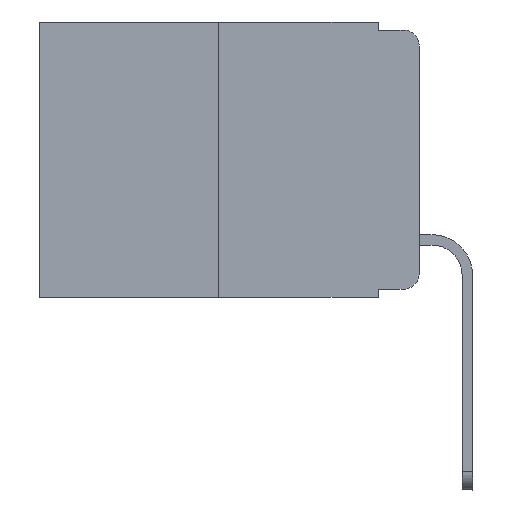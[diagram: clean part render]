
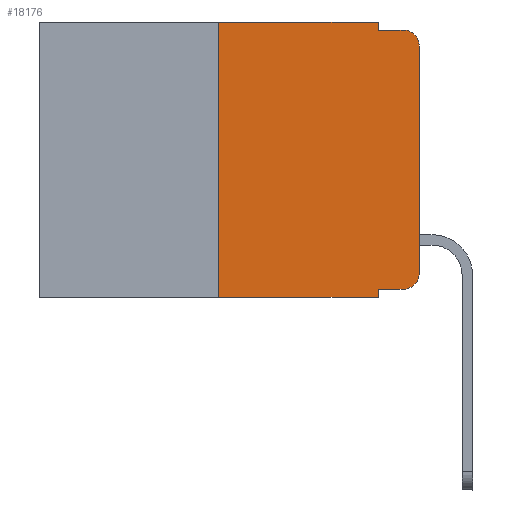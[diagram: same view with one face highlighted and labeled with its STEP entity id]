
A CAD part, left-side view. The second image highlights one B-rep face of the part: STEP entity #18176.
In plain terms, the highlighted planar face has unit normal (-1, 0, 0).
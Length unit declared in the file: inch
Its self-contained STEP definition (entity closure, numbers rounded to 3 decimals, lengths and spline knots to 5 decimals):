
#63 = LINE ( 'NONE', #7052, #14666 ) ;
#671 = EDGE_CURVE ( 'NONE', #14336, #9487, #5122, .T. ) ;
#809 = CARTESIAN_POINT ( 'NONE',  ( 0., 0.051, -0.01 ) ) ;
#1012 = AXIS2_PLACEMENT_3D ( 'NONE', #3550, #15054, #13811 ) ;
#1521 = EDGE_CURVE ( 'NONE', #14336, #9455, #9280, .T. ) ;
#2181 = CARTESIAN_POINT ( 'NONE',  ( 0., 0.473, -0.343 ) ) ;
#2260 = CARTESIAN_POINT ( 'NONE',  ( 0., 0.25, 0. ) ) ;
#2397 = EDGE_CURVE ( 'NONE', #13521, #18033, #18646, .T. ) ;
#2417 = CARTESIAN_POINT ( 'NONE',  ( 0., 0.02, -0.313 ) ) ;
#2476 = EDGE_CURVE ( 'NONE', #17727, #13521, #7102, .T. ) ;
#2742 = DIRECTION ( 'NONE',  ( 0., 0., -1. ) ) ;
#3067 = CARTESIAN_POINT ( 'NONE',  ( 0., 0., 0. ) ) ;
#3352 = CARTESIAN_POINT ( 'NONE',  ( 0., 0.02, -0.03 ) ) ;
#3537 = ORIENTED_EDGE ( 'NONE', *, *, #671, .F. ) ;
#3550 = CARTESIAN_POINT ( 'NONE',  ( 0., 0.473, 0. ) ) ;
#3731 = CIRCLE ( 'NONE', #13853, 0.02 ) ;
#3777 = VERTEX_POINT ( 'NONE', #18814 ) ;
#4081 = CARTESIAN_POINT ( 'NONE',  ( 0., 0.473, 0. ) ) ;
#4153 = VERTEX_POINT ( 'NONE', #14195 ) ;
#4669 = CARTESIAN_POINT ( 'NONE',  ( 0., 0.25, -0.343 ) ) ;
#4713 = ORIENTED_EDGE ( 'NONE', *, *, #2397, .F. ) ;
#4789 = DIRECTION ( 'NONE',  ( -1., 0., 0. ) ) ;
#5072 = ORIENTED_EDGE ( 'NONE', *, *, #10056, .T. ) ;
#5122 = LINE ( 'NONE', #2260, #18794 ) ;
#5195 = DIRECTION ( 'NONE',  ( 0., 0., -1. ) ) ;
#5305 = DIRECTION ( 'NONE',  ( 0., -1., 0. ) ) ;
#5473 = ORIENTED_EDGE ( 'NONE', *, *, #10924, .T. ) ;
#5514 = LINE ( 'NONE', #3067, #11443 ) ;
#5567 = CARTESIAN_POINT ( 'NONE',  ( 0., 0., -0.313 ) ) ;
#6349 = DIRECTION ( 'NONE',  ( 0., 0., 1. ) ) ;
#6787 = LINE ( 'NONE', #11323, #15394 ) ;
#6829 = DIRECTION ( 'NONE',  ( 0., 0., -1. ) ) ;
#7052 = CARTESIAN_POINT ( 'NONE',  ( 0., 0.051, 0. ) ) ;
#7102 = LINE ( 'NONE', #12617, #8532 ) ;
#7845 = FACE_OUTER_BOUND ( 'NONE', #18518, .T. ) ;
#8532 = VECTOR ( 'NONE', #5195, 39.37008 ) ;
#8569 = DIRECTION ( 'NONE',  ( 0., -1., 0. ) ) ;
#9200 = PLANE ( 'NONE',  #1012 ) ;
#9280 = LINE ( 'NONE', #2181, #13038 ) ;
#9404 = DIRECTION ( 'NONE',  ( 0., 0., -1. ) ) ;
#9455 = VERTEX_POINT ( 'NONE', #15038 ) ;
#9487 = VERTEX_POINT ( 'NONE', #12475 ) ;
#9656 = CARTESIAN_POINT ( 'NONE',  ( 0., 0.051, -0.333 ) ) ;
#9951 = VERTEX_POINT ( 'NONE', #9656 ) ;
#10056 = EDGE_CURVE ( 'NONE', #16445, #4153, #5514, .T. ) ;
#10081 = EDGE_CURVE ( 'NONE', #9487, #17727, #17662, .T. ) ;
#10394 = CIRCLE ( 'NONE', #11640, 0.02 ) ;
#10924 = EDGE_CURVE ( 'NONE', #9951, #3777, #6787, .T. ) ;
#11323 = CARTESIAN_POINT ( 'NONE',  ( 0., 0.051, -0.333 ) ) ;
#11443 = VECTOR ( 'NONE', #14262, 39.37008 ) ;
#11640 = AXIS2_PLACEMENT_3D ( 'NONE', #3352, #4789, #9404 ) ;
#12182 = ORIENTED_EDGE ( 'NONE', *, *, #10081, .F. ) ;
#12469 = DIRECTION ( 'NONE',  ( 0., -1., 0. ) ) ;
#12475 = CARTESIAN_POINT ( 'NONE',  ( 0., 0.25, 0. ) ) ;
#12490 = CARTESIAN_POINT ( 'NONE',  ( 0., 0.02, -0.01 ) ) ;
#12522 = ORIENTED_EDGE ( 'NONE', *, *, #14741, .F. ) ;
#12617 = CARTESIAN_POINT ( 'NONE',  ( 0., 0.051, 0. ) ) ;
#13038 = VECTOR ( 'NONE', #12469, 39.37008 ) ;
#13521 = VERTEX_POINT ( 'NONE', #809 ) ;
#13811 = DIRECTION ( 'NONE',  ( 0., 0., -1. ) ) ;
#13853 = AXIS2_PLACEMENT_3D ( 'NONE', #2417, #18828, #6829 ) ;
#13947 = CARTESIAN_POINT ( 'NONE',  ( 0., 0.051, 0. ) ) ;
#14195 = CARTESIAN_POINT ( 'NONE',  ( 0., 0., -0.03 ) ) ;
#14262 = DIRECTION ( 'NONE',  ( 0., 0., 1. ) ) ;
#14336 = VERTEX_POINT ( 'NONE', #4669 ) ;
#14666 = VECTOR ( 'NONE', #2742, 39.37008 ) ;
#14741 = EDGE_CURVE ( 'NONE', #9951, #9455, #63, .T. ) ;
#15038 = CARTESIAN_POINT ( 'NONE',  ( 0., 0.051, -0.343 ) ) ;
#15054 = DIRECTION ( 'NONE',  ( 1., 0., 0. ) ) ;
#15333 = EDGE_CURVE ( 'NONE', #4153, #18033, #10394, .T. ) ;
#15394 = VECTOR ( 'NONE', #18697, 39.37008 ) ;
#15612 = VECTOR ( 'NONE', #5305, 39.37008 ) ;
#15861 = ORIENTED_EDGE ( 'NONE', *, *, #1521, .T. ) ;
#16445 = VERTEX_POINT ( 'NONE', #5567 ) ;
#17190 = ORIENTED_EDGE ( 'NONE', *, *, #2476, .F. ) ;
#17662 = LINE ( 'NONE', #4081, #18442 ) ;
#17727 = VERTEX_POINT ( 'NONE', #13947 ) ;
#17729 = ORIENTED_EDGE ( 'NONE', *, *, #15333, .T. ) ;
#17797 = EDGE_CURVE ( 'NONE', #3777, #16445, #3731, .T. ) ;
#18033 = VERTEX_POINT ( 'NONE', #12490 ) ;
#18176 = ADVANCED_FACE ( 'NONE', ( #7845 ), #9200, .F. ) ;
#18442 = VECTOR ( 'NONE', #8569, 39.37008 ) ;
#18518 = EDGE_LOOP ( 'NONE', ( #5072, #17729, #4713, #17190, #12182, #3537, #15861, #12522, #5473, #18787 ) ) ;
#18646 = LINE ( 'NONE', #18735, #15612 ) ;
#18697 = DIRECTION ( 'NONE',  ( 0., -1., 0. ) ) ;
#18735 = CARTESIAN_POINT ( 'NONE',  ( 0., 0.051, -0.01 ) ) ;
#18787 = ORIENTED_EDGE ( 'NONE', *, *, #17797, .T. ) ;
#18794 = VECTOR ( 'NONE', #6349, 39.37008 ) ;
#18814 = CARTESIAN_POINT ( 'NONE',  ( 0., 0.02, -0.333 ) ) ;
#18828 = DIRECTION ( 'NONE',  ( -1., 0., 0. ) ) ;
